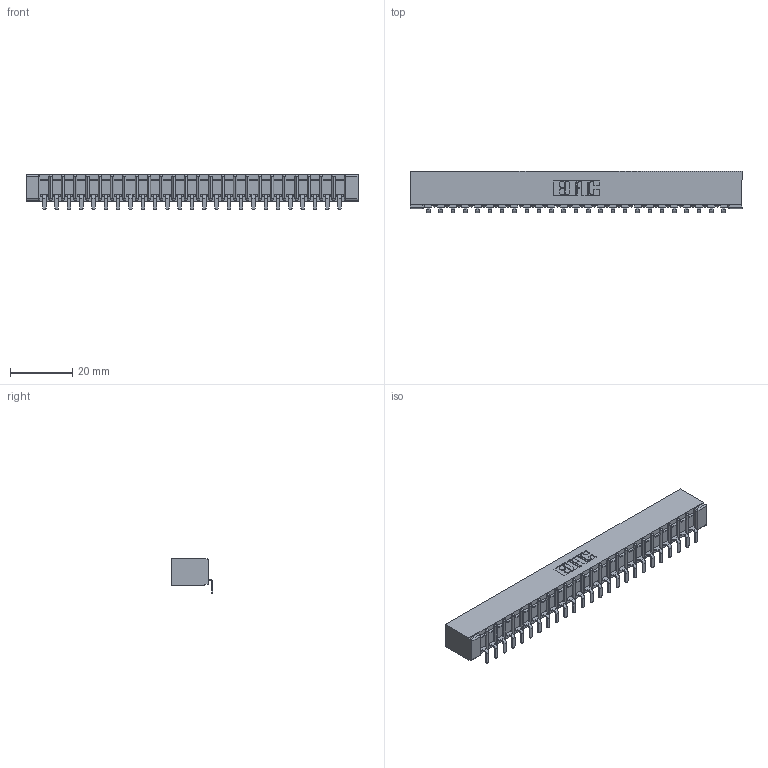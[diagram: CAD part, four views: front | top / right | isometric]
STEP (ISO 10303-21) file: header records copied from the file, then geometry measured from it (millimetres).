
FILE_DESCRIPTION (( 'STEP AP203' ), '1' );
FILE_NAME ('357-025-553-101.STEP', '2019-09-17T00:40:44', ( '' ), ( '' ), 'SwSTEP 2.0', 'SolidWorks 2016', '' );
FILE_SCHEMA (( 'CONFIG_CONTROL_DESIGN' ));
Length unit declared in the file: inch
Products named in the file (3): 357-025-553-101; 307-290-002_553; 307 Part_No Mounting Lugs
Assembly tree (26 placements, depth 2):
  357-025-553-101
    307 Part_No Mounting Lugs
    307-290-002_553  x25
Bounding box: 106.93 x 13.32 x 11.51 mm (x, y, z)
Volume: 7303.3 mm3; surface area: 13965.1 mm2
Topology: 26 solids, 26 shells, 2086 faces, 6399 edges, 4194 vertices
Faces by surface type: plane 1241, cylinder 793, sphere 52
Entity records: 24104 total; most frequent: CARTESIAN_POINT 4064, ORIENTED_EDGE 4054, DIRECTION 3955, EDGE_CURVE 2027, VECTOR 1545, LINE 1545, VERTEX_POINT 1314, AXIS2_PLACEMENT_3D 1205
